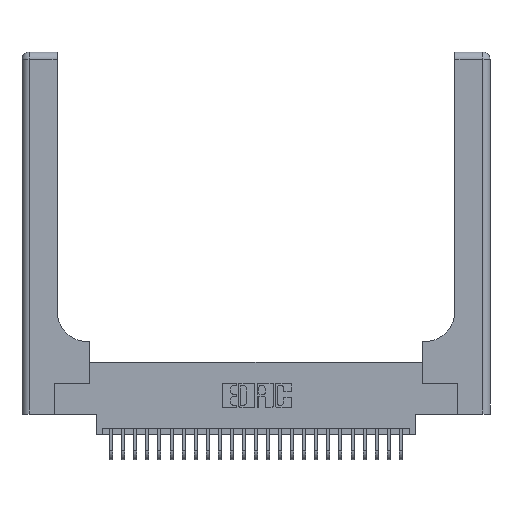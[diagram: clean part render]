
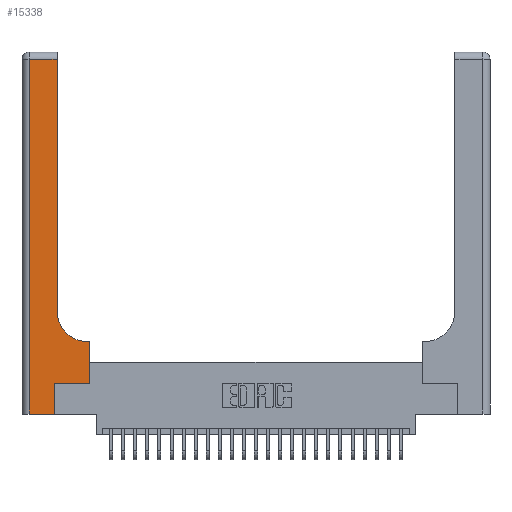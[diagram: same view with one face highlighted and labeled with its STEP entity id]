
A CAD part, top view. The second image highlights one B-rep face of the part: STEP entity #15338.
In plain terms, the highlighted planar face has unit normal (0, 0, 1).
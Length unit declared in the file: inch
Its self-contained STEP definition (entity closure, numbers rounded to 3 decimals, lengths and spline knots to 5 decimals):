
#351 = ORIENTED_EDGE ( 'NONE', *, *, #23452, .T. ) ;
#556 = VECTOR ( 'NONE', #25146, 39.37008 ) ;
#668 = VERTEX_POINT ( 'NONE', #19301 ) ;
#928 = AXIS2_PLACEMENT_3D ( 'NONE', #16780, #3414, #19045 ) ;
#2290 = CARTESIAN_POINT ( 'NONE',  ( 0., 2.94, 0.37 ) ) ;
#3414 = DIRECTION ( 'NONE',  ( 0., 0., -1. ) ) ;
#3810 = DIRECTION ( 'NONE',  ( 0., 1., 0. ) ) ;
#3846 = DIRECTION ( 'NONE',  ( 1., 0., 0. ) ) ;
#3939 = ORIENTED_EDGE ( 'NONE', *, *, #21724, .T. ) ;
#4471 = CARTESIAN_POINT ( 'NONE',  ( 0.5585, 0.6, 0.37 ) ) ;
#5222 = EDGE_LOOP ( 'NONE', ( #21362, #3939, #22553, #12593, #351, #21192, #12783, #23894, #17923 ) ) ;
#5252 = CARTESIAN_POINT ( 'NONE',  ( 0.269, 0.25, 0.37 ) ) ;
#5709 = CARTESIAN_POINT ( 'NONE',  ( 0.5585, 0.25, 0.37 ) ) ;
#6007 = CARTESIAN_POINT ( 'NONE',  ( 0., 3., 0.37 ) ) ;
#6080 = CARTESIAN_POINT ( 'NONE',  ( 0.269, 0., 0.37 ) ) ;
#6081 = CARTESIAN_POINT ( 'NONE',  ( 0.5585, 0.25, 0.37 ) ) ;
#6951 = VECTOR ( 'NONE', #15666, 39.37008 ) ;
#7287 = VERTEX_POINT ( 'NONE', #21495 ) ;
#7324 = CARTESIAN_POINT ( 'NONE',  ( 0.269, 0., 0.37 ) ) ;
#7380 = VERTEX_POINT ( 'NONE', #6080 ) ;
#7465 = CARTESIAN_POINT ( 'NONE',  ( 0.06, 3., 0.37 ) ) ;
#8257 = VECTOR ( 'NONE', #20955, 39.37008 ) ;
#8764 = CIRCLE ( 'NONE', #928, 0.25 ) ;
#9540 = DIRECTION ( 'NONE',  ( -1., 0., 0. ) ) ;
#10297 = VERTEX_POINT ( 'NONE', #27276 ) ;
#10322 = FACE_OUTER_BOUND ( 'NONE', #5222, .T. ) ;
#11014 = LINE ( 'NONE', #7324, #556 ) ;
#11938 = VERTEX_POINT ( 'NONE', #5709 ) ;
#12229 = VECTOR ( 'NONE', #3810, 39.37008 ) ;
#12593 = ORIENTED_EDGE ( 'NONE', *, *, #27725, .T. ) ;
#12726 = DIRECTION ( 'NONE',  ( -1., 0., 0. ) ) ;
#12783 = ORIENTED_EDGE ( 'NONE', *, *, #24447, .T. ) ;
#12809 = DIRECTION ( 'NONE',  ( 0., 1., 0. ) ) ;
#12879 = LINE ( 'NONE', #2290, #6951 ) ;
#13635 = VERTEX_POINT ( 'NONE', #25971 ) ;
#14078 = DIRECTION ( 'NONE',  ( 0., -1., 0. ) ) ;
#14863 = LINE ( 'NONE', #5252, #8257 ) ;
#14926 = VERTEX_POINT ( 'NONE', #4471 ) ;
#14935 = CARTESIAN_POINT ( 'NONE',  ( 0.2915, 3., 0.37 ) ) ;
#15338 = ADVANCED_FACE ( 'NONE', ( #10322 ), #19369, .F. ) ;
#15477 = CARTESIAN_POINT ( 'NONE',  ( 0.269, 0.25, 0.37 ) ) ;
#15666 = DIRECTION ( 'NONE',  ( -1., 0., 0. ) ) ;
#16269 = VECTOR ( 'NONE', #9540, 39.37008 ) ;
#16444 = CARTESIAN_POINT ( 'NONE',  ( 0.06, 2.94, 0.37 ) ) ;
#16780 = CARTESIAN_POINT ( 'NONE',  ( 0.5415, 0.85, 0.37 ) ) ;
#16952 = LINE ( 'NONE', #20667, #16269 ) ;
#17038 = VECTOR ( 'NONE', #3846, 39.37008 ) ;
#17203 = CARTESIAN_POINT ( 'NONE',  ( 0., 0., 0.37 ) ) ;
#17798 = VERTEX_POINT ( 'NONE', #16444 ) ;
#17923 = ORIENTED_EDGE ( 'NONE', *, *, #26380, .T. ) ;
#18364 = EDGE_CURVE ( 'NONE', #17798, #13635, #26893, .T. ) ;
#18875 = LINE ( 'NONE', #14935, #12229 ) ;
#19045 = DIRECTION ( 'NONE',  ( 1., 0., 0. ) ) ;
#19301 = CARTESIAN_POINT ( 'NONE',  ( 0.5415, 0.6, 0.37 ) ) ;
#19345 = VERTEX_POINT ( 'NONE', #15477 ) ;
#19369 = PLANE ( 'NONE',  #21871 ) ;
#20667 = CARTESIAN_POINT ( 'NONE',  ( 0.2915, 0.6, 0.37 ) ) ;
#20753 = LINE ( 'NONE', #6081, #25274 ) ;
#20955 = DIRECTION ( 'NONE',  ( 1., 0., 0. ) ) ;
#21192 = ORIENTED_EDGE ( 'NONE', *, *, #23526, .T. ) ;
#21362 = ORIENTED_EDGE ( 'NONE', *, *, #26495, .T. ) ;
#21495 = CARTESIAN_POINT ( 'NONE',  ( 0.2915, 2.94, 0.37 ) ) ;
#21724 = EDGE_CURVE ( 'NONE', #7287, #17798, #12879, .T. ) ;
#21871 = AXIS2_PLACEMENT_3D ( 'NONE', #6007, #26082, #12726 ) ;
#22281 = LINE ( 'NONE', #17203, #17038 ) ;
#22553 = ORIENTED_EDGE ( 'NONE', *, *, #18364, .T. ) ;
#23441 = EDGE_CURVE ( 'NONE', #14926, #668, #16952, .T. ) ;
#23452 = EDGE_CURVE ( 'NONE', #7380, #19345, #11014, .T. ) ;
#23526 = EDGE_CURVE ( 'NONE', #19345, #11938, #14863, .T. ) ;
#23894 = ORIENTED_EDGE ( 'NONE', *, *, #23441, .T. ) ;
#24447 = EDGE_CURVE ( 'NONE', #11938, #14926, #20753, .T. ) ;
#25146 = DIRECTION ( 'NONE',  ( 0., 1., 0. ) ) ;
#25274 = VECTOR ( 'NONE', #12809, 39.37008 ) ;
#25971 = CARTESIAN_POINT ( 'NONE',  ( 0.06, 0., 0.37 ) ) ;
#26082 = DIRECTION ( 'NONE',  ( 0., 0., -1. ) ) ;
#26380 = EDGE_CURVE ( 'NONE', #668, #10297, #8764, .T. ) ;
#26495 = EDGE_CURVE ( 'NONE', #10297, #7287, #18875, .T. ) ;
#26893 = LINE ( 'NONE', #7465, #27608 ) ;
#27276 = CARTESIAN_POINT ( 'NONE',  ( 0.2915, 0.85, 0.37 ) ) ;
#27608 = VECTOR ( 'NONE', #14078, 39.37008 ) ;
#27725 = EDGE_CURVE ( 'NONE', #13635, #7380, #22281, .T. ) ;
